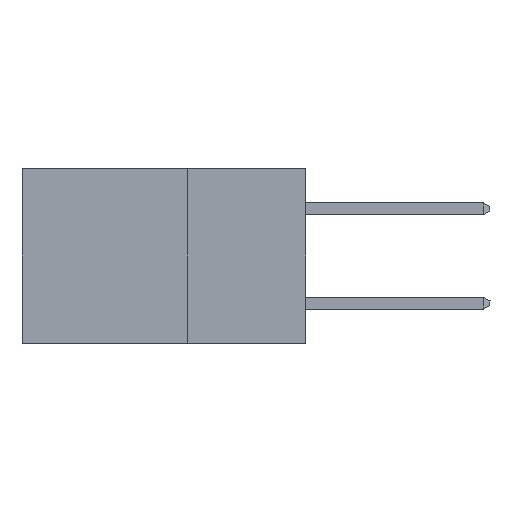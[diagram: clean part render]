
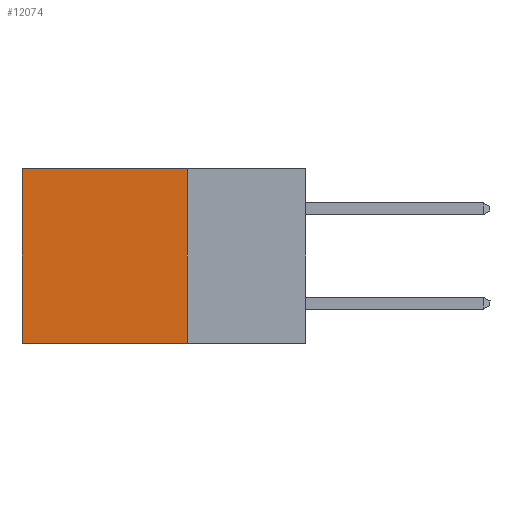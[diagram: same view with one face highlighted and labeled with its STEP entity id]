
A CAD part, left-side view. The second image highlights one B-rep face of the part: STEP entity #12074.
In plain terms, the highlighted planar face has unit normal (-1, 0, 0).
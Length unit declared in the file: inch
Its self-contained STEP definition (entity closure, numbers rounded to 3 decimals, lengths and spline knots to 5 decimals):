
#17 = DIRECTION ( 'NONE',  ( 0., 0., -1. ) ) ;
#482 = EDGE_CURVE ( 'NONE', #1165, #13524, #17327, .T. ) ;
#529 = ORIENTED_EDGE ( 'NONE', *, *, #482, .F. ) ;
#835 = CARTESIAN_POINT ( 'NONE',  ( 0.298, 0.6, -0.37 ) ) ;
#1080 = DIRECTION ( 'NONE',  ( 0., 1., 0. ) ) ;
#1165 = VERTEX_POINT ( 'NONE', #11834 ) ;
#1239 = VECTOR ( 'NONE', #1080, 39.37008 ) ;
#1299 = CARTESIAN_POINT ( 'NONE',  ( 0.298, 0.6, 0. ) ) ;
#1689 = CARTESIAN_POINT ( 'NONE',  ( 0.298, 0.25, -0.37 ) ) ;
#1693 = LINE ( 'NONE', #11478, #1239 ) ;
#3674 = LINE ( 'NONE', #18227, #4370 ) ;
#4242 = CARTESIAN_POINT ( 'NONE',  ( 0.298, 0.25, -0.37 ) ) ;
#4370 = VECTOR ( 'NONE', #4958, 39.37008 ) ;
#4958 = DIRECTION ( 'NONE',  ( 0., 0., -1. ) ) ;
#5276 = EDGE_LOOP ( 'NONE', ( #15885, #9708, #529, #12409 ) ) ;
#6020 = PLANE ( 'NONE',  #12871 ) ;
#7384 = VERTEX_POINT ( 'NONE', #1299 ) ;
#8347 = VECTOR ( 'NONE', #13078, 39.37008 ) ;
#8605 = EDGE_CURVE ( 'NONE', #1165, #7384, #1693, .T. ) ;
#9326 = EDGE_CURVE ( 'NONE', #13524, #11810, #14305, .T. ) ;
#9708 = ORIENTED_EDGE ( 'NONE', *, *, #9326, .F. ) ;
#11478 = CARTESIAN_POINT ( 'NONE',  ( 0.298, 0.25, 0. ) ) ;
#11484 = DIRECTION ( 'NONE',  ( 0., 0., -1. ) ) ;
#11810 = VERTEX_POINT ( 'NONE', #835 ) ;
#11834 = CARTESIAN_POINT ( 'NONE',  ( 0.298, 0.25, 0. ) ) ;
#12074 = ADVANCED_FACE ( 'NONE', ( #12277 ), #6020, .F. ) ;
#12277 = FACE_OUTER_BOUND ( 'NONE', #5276, .T. ) ;
#12409 = ORIENTED_EDGE ( 'NONE', *, *, #8605, .T. ) ;
#12871 = AXIS2_PLACEMENT_3D ( 'NONE', #18920, #16338, #17 ) ;
#13078 = DIRECTION ( 'NONE',  ( 0., 1., 0. ) ) ;
#13524 = VERTEX_POINT ( 'NONE', #1689 ) ;
#13588 = EDGE_CURVE ( 'NONE', #7384, #11810, #3674, .T. ) ;
#14031 = CARTESIAN_POINT ( 'NONE',  ( 0.298, 0.25, 0. ) ) ;
#14151 = VECTOR ( 'NONE', #11484, 39.37008 ) ;
#14305 = LINE ( 'NONE', #4242, #8347 ) ;
#15885 = ORIENTED_EDGE ( 'NONE', *, *, #13588, .T. ) ;
#16338 = DIRECTION ( 'NONE',  ( 1., 0., 0. ) ) ;
#17327 = LINE ( 'NONE', #14031, #14151 ) ;
#18227 = CARTESIAN_POINT ( 'NONE',  ( 0.298, 0.6, 0. ) ) ;
#18920 = CARTESIAN_POINT ( 'NONE',  ( 0.298, 0.25, 0. ) ) ;
